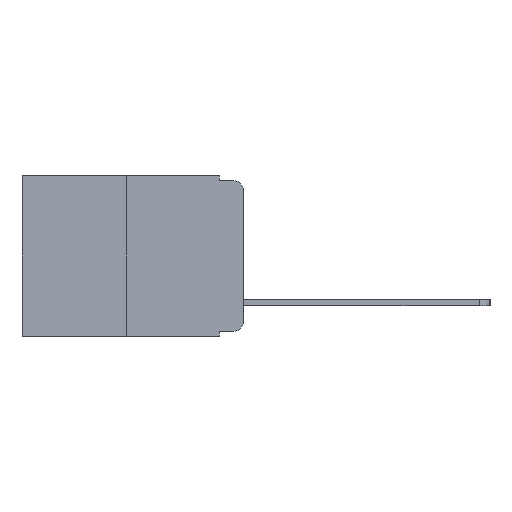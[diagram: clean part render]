
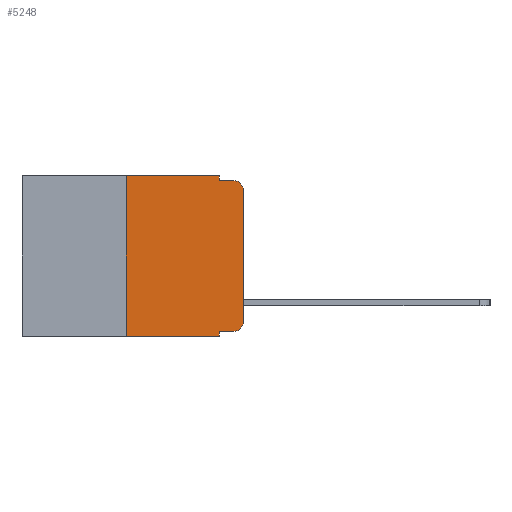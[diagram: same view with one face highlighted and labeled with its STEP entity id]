
A CAD part, left-side view. The second image highlights one B-rep face of the part: STEP entity #5248.
In plain terms, the highlighted planar face has unit normal (-1, 0, 0).
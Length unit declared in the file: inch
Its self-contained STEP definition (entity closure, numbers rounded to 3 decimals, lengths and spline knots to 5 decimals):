
#815 = VERTEX_POINT ( 'NONE', #7590 ) ;
#935 = ORIENTED_EDGE ( 'NONE', *, *, #6653, .T. ) ;
#961 = CARTESIAN_POINT ( 'NONE',  ( 0., 0.051, 0. ) ) ;
#969 = LINE ( 'NONE', #16988, #10568 ) ;
#1343 = CARTESIAN_POINT ( 'NONE',  ( 0., 0.051, -0.01 ) ) ;
#1480 = EDGE_CURVE ( 'NONE', #24108, #21294, #4293, .T. ) ;
#1551 = VECTOR ( 'NONE', #21036, 39.37008 ) ;
#1571 = VECTOR ( 'NONE', #22483, 39.37008 ) ;
#2197 = LINE ( 'NONE', #18758, #1571 ) ;
#2802 = EDGE_CURVE ( 'NONE', #21294, #3152, #5758, .T. ) ;
#3127 = CARTESIAN_POINT ( 'NONE',  ( 0., 0.051, -0.343 ) ) ;
#3152 = VERTEX_POINT ( 'NONE', #9804 ) ;
#3269 = VERTEX_POINT ( 'NONE', #23194 ) ;
#3300 = AXIS2_PLACEMENT_3D ( 'NONE', #16119, #4796, #17961 ) ;
#3509 = EDGE_LOOP ( 'NONE', ( #11643, #21809, #21768, #15521, #13712, #13735, #17627, #9604, #935, #4210 ) ) ;
#3619 = CIRCLE ( 'NONE', #19979, 0.02 ) ;
#4087 = EDGE_CURVE ( 'NONE', #20997, #3152, #15694, .T. ) ;
#4178 = CARTESIAN_POINT ( 'NONE',  ( 0., 0.473, 0. ) ) ;
#4210 = ORIENTED_EDGE ( 'NONE', *, *, #10438, .T. ) ;
#4293 = LINE ( 'NONE', #7490, #22500 ) ;
#4756 = PLANE ( 'NONE',  #10516 ) ;
#4796 = DIRECTION ( 'NONE',  ( -1., 0., 0. ) ) ;
#5248 = ADVANCED_FACE ( 'NONE', ( #9783 ), #4756, .F. ) ;
#5401 = EDGE_CURVE ( 'NONE', #10937, #20997, #21115, .T. ) ;
#5758 = CIRCLE ( 'NONE', #3300, 0.02 ) ;
#6092 = CARTESIAN_POINT ( 'NONE',  ( 0., 0.473, -0.343 ) ) ;
#6125 = LINE ( 'NONE', #6092, #1551 ) ;
#6653 = EDGE_CURVE ( 'NONE', #3269, #17126, #2197, .T. ) ;
#6693 = EDGE_CURVE ( 'NONE', #815, #11754, #969, .T. ) ;
#6760 = VECTOR ( 'NONE', #23519, 39.37008 ) ;
#6831 = EDGE_CURVE ( 'NONE', #11754, #10937, #13208, .T. ) ;
#7126 = DIRECTION ( 'NONE',  ( 0., -1., 0. ) ) ;
#7490 = CARTESIAN_POINT ( 'NONE',  ( 0., 0., 0. ) ) ;
#7590 = CARTESIAN_POINT ( 'NONE',  ( 0., 0.25, -0.343 ) ) ;
#7620 = VECTOR ( 'NONE', #21082, 39.37008 ) ;
#8520 = DIRECTION ( 'NONE',  ( -1., 0., 0. ) ) ;
#9604 = ORIENTED_EDGE ( 'NONE', *, *, #20324, .F. ) ;
#9783 = FACE_OUTER_BOUND ( 'NONE', #3509, .T. ) ;
#9804 = CARTESIAN_POINT ( 'NONE',  ( 0., 0.02, -0.01 ) ) ;
#10438 = EDGE_CURVE ( 'NONE', #17126, #24108, #3619, .T. ) ;
#10507 = DIRECTION ( 'NONE',  ( 0., 0., -1. ) ) ;
#10516 = AXIS2_PLACEMENT_3D ( 'NONE', #21572, #21657, #10507 ) ;
#10568 = VECTOR ( 'NONE', #24420, 39.37008 ) ;
#10665 = CARTESIAN_POINT ( 'NONE',  ( 0., 0.25, 0. ) ) ;
#10937 = VERTEX_POINT ( 'NONE', #12028 ) ;
#11245 = VECTOR ( 'NONE', #20277, 39.37008 ) ;
#11643 = ORIENTED_EDGE ( 'NONE', *, *, #1480, .T. ) ;
#11754 = VERTEX_POINT ( 'NONE', #10665 ) ;
#12028 = CARTESIAN_POINT ( 'NONE',  ( 0., 0.051, 0. ) ) ;
#13208 = LINE ( 'NONE', #4178, #7620 ) ;
#13712 = ORIENTED_EDGE ( 'NONE', *, *, #6831, .F. ) ;
#13735 = ORIENTED_EDGE ( 'NONE', *, *, #6693, .F. ) ;
#14666 = EDGE_CURVE ( 'NONE', #815, #17921, #6125, .T. ) ;
#15521 = ORIENTED_EDGE ( 'NONE', *, *, #5401, .F. ) ;
#15694 = LINE ( 'NONE', #1343, #19442 ) ;
#16119 = CARTESIAN_POINT ( 'NONE',  ( 0., 0.02, -0.03 ) ) ;
#16988 = CARTESIAN_POINT ( 'NONE',  ( 0., 0.25, 0. ) ) ;
#17126 = VERTEX_POINT ( 'NONE', #23258 ) ;
#17627 = ORIENTED_EDGE ( 'NONE', *, *, #14666, .T. ) ;
#17921 = VERTEX_POINT ( 'NONE', #3127 ) ;
#17961 = DIRECTION ( 'NONE',  ( 0., 0., -1. ) ) ;
#18411 = CARTESIAN_POINT ( 'NONE',  ( 0., 0.051, 0. ) ) ;
#18687 = DIRECTION ( 'NONE',  ( 0., 0., 1. ) ) ;
#18758 = CARTESIAN_POINT ( 'NONE',  ( 0., 0.051, -0.333 ) ) ;
#19442 = VECTOR ( 'NONE', #7126, 39.37008 ) ;
#19673 = CARTESIAN_POINT ( 'NONE',  ( 0., 0.02, -0.313 ) ) ;
#19979 = AXIS2_PLACEMENT_3D ( 'NONE', #19673, #8520, #21528 ) ;
#20277 = DIRECTION ( 'NONE',  ( 0., 0., -1. ) ) ;
#20324 = EDGE_CURVE ( 'NONE', #3269, #17921, #21644, .T. ) ;
#20466 = CARTESIAN_POINT ( 'NONE',  ( 0., 0., -0.313 ) ) ;
#20997 = VERTEX_POINT ( 'NONE', #23905 ) ;
#21036 = DIRECTION ( 'NONE',  ( 0., -1., 0. ) ) ;
#21082 = DIRECTION ( 'NONE',  ( 0., -1., 0. ) ) ;
#21115 = LINE ( 'NONE', #18411, #11245 ) ;
#21294 = VERTEX_POINT ( 'NONE', #22987 ) ;
#21528 = DIRECTION ( 'NONE',  ( 0., 0., -1. ) ) ;
#21572 = CARTESIAN_POINT ( 'NONE',  ( 0., 0.473, 0. ) ) ;
#21644 = LINE ( 'NONE', #961, #6760 ) ;
#21657 = DIRECTION ( 'NONE',  ( 1., 0., 0. ) ) ;
#21768 = ORIENTED_EDGE ( 'NONE', *, *, #4087, .F. ) ;
#21809 = ORIENTED_EDGE ( 'NONE', *, *, #2802, .T. ) ;
#22483 = DIRECTION ( 'NONE',  ( 0., -1., 0. ) ) ;
#22500 = VECTOR ( 'NONE', #18687, 39.37008 ) ;
#22987 = CARTESIAN_POINT ( 'NONE',  ( 0., 0., -0.03 ) ) ;
#23194 = CARTESIAN_POINT ( 'NONE',  ( 0., 0.051, -0.333 ) ) ;
#23258 = CARTESIAN_POINT ( 'NONE',  ( 0., 0.02, -0.333 ) ) ;
#23519 = DIRECTION ( 'NONE',  ( 0., 0., -1. ) ) ;
#23905 = CARTESIAN_POINT ( 'NONE',  ( 0., 0.051, -0.01 ) ) ;
#24108 = VERTEX_POINT ( 'NONE', #20466 ) ;
#24420 = DIRECTION ( 'NONE',  ( 0., 0., 1. ) ) ;
